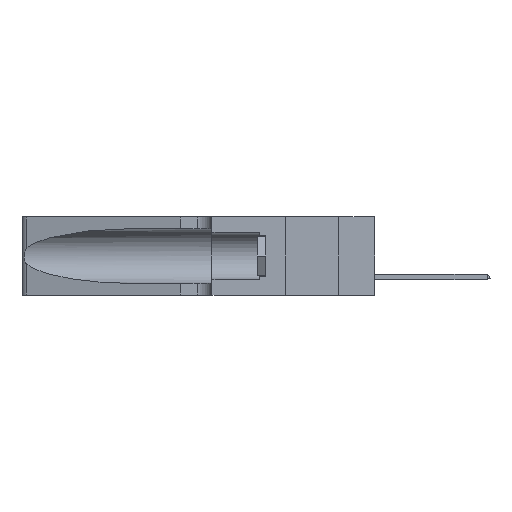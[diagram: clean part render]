
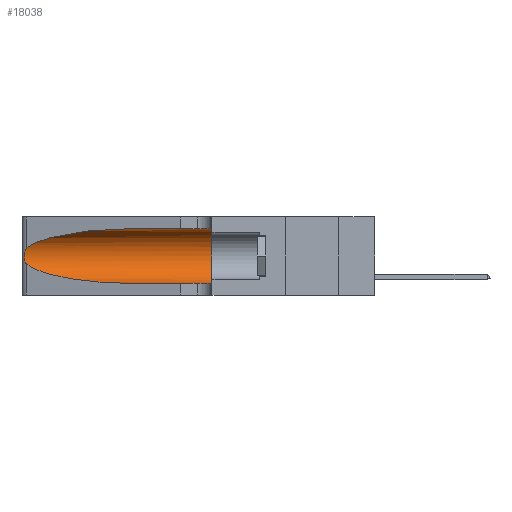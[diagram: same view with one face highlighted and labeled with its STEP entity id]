
A CAD part, left-side view. The second image highlights one B-rep face of the part: STEP entity #18038.
In plain terms, the highlighted cylindrical face has radius 3.308 mm (diameter 6.617 mm), a partial arc.
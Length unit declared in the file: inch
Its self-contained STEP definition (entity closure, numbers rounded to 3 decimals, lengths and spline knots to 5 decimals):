
#144 = CARTESIAN_POINT ( 'NONE',  ( 0.18966, 0.96281, 0.05475 ) ) ;
#435 = ORIENTED_EDGE ( 'NONE', *, *, #25085, .T. ) ;
#989 = CARTESIAN_POINT ( 'NONE',  ( 0.25787, 1.23484, 0.2124 ) ) ;
#1085 = CARTESIAN_POINT ( 'NONE',  ( 0.25487, 1.22718, 0.22369 ) ) ;
#1579 = DIRECTION ( 'NONE',  ( 0., -1., 0. ) ) ;
#2005 = ORIENTED_EDGE ( 'NONE', *, *, #19564, .T. ) ;
#2217 = CARTESIAN_POINT ( 'NONE',  ( 0.25487, 1.22718, 0.22369 ) ) ;
#2556 =( BOUNDED_CURVE ( )  B_SPLINE_CURVE ( 3, ( #8768, #8676, #17354, #2217 ),
 .UNSPECIFIED., .F., .F. ) 
 B_SPLINE_CURVE_WITH_KNOTS ( ( 4, 4 ),
 ( 1.5708, 2.84003 ),
 .UNSPECIFIED. ) 
 CURVE ( )  GEOMETRIC_REPRESENTATION_ITEM ( )  RATIONAL_B_SPLINE_CURVE ( ( 1., 0.87, 0.87, 1. ) ) 
 REPRESENTATION_ITEM ( '' )  );
#2606 = CARTESIAN_POINT ( 'NONE',  ( 0.1305, 0.35, 0.31525 ) ) ;
#3124 = CARTESIAN_POINT ( 'NONE',  ( 0.25487, 1.22718, 0.14631 ) ) ;
#3735 = CIRCLE ( 'NONE', #20630, 0.13025 ) ;
#3801 = CARTESIAN_POINT ( 'NONE',  ( 0.1305, 0.35, 0.05475 ) ) ;
#4142 = CARTESIAN_POINT ( 'NONE',  ( 0.1305, 1.61858, 0.05475 ) ) ;
#5543 = CARTESIAN_POINT ( 'NONE',  ( 0.26075, 1.23896, 0.19203 ) ) ;
#6054 = VECTOR ( 'NONE', #19007, 39.37008 ) ;
#6077 = EDGE_CURVE ( 'NONE', #18598, #22260, #2556, .T. ) ;
#6341 = CARTESIAN_POINT ( 'NONE',  ( 0.1305, 0.72297, 0.05475 ) ) ;
#6590 = CARTESIAN_POINT ( 'NONE',  ( 0.1305, 0.72297, 0.05475 ) ) ;
#6756 = CYLINDRICAL_SURFACE ( 'NONE', #26014, 0.13025 ) ;
#6841 = B_SPLINE_CURVE_WITH_KNOTS ( 'NONE', 3,
 ( #1085, #26986, #11624, #989, #11719, #15912, #5543, #13962, #26617, #7710, #26910, #9582, #18256, #3124 ),
 .UNSPECIFIED., .F., .F.,
 ( 4, 2, 2, 2, 2, 2, 4 ),
 ( 0., 0.00027, 0.00053, 0.00107, 0.0016, 0.00187, 0.00214 ),
 .UNSPECIFIED. ) ;
#7710 = CARTESIAN_POINT ( 'NONE',  ( 0.25856, 1.23593, 0.16098 ) ) ;
#7820 = CARTESIAN_POINT ( 'NONE',  ( 0.1305, 0.35, 0.185 ) ) ;
#8245 = EDGE_LOOP ( 'NONE', ( #21621, #435, #2005, #24810, #24538, #18217 ) ) ;
#8676 = CARTESIAN_POINT ( 'NONE',  ( 0.18966, 0.96281, 0.31525 ) ) ;
#8768 = CARTESIAN_POINT ( 'NONE',  ( 0.1305, 0.72297, 0.31525 ) ) ;
#9091 = LINE ( 'NONE', #4142, #6054 ) ;
#9095 = FACE_OUTER_BOUND ( 'NONE', #8245, .T. ) ;
#9199 = CARTESIAN_POINT ( 'NONE',  ( 0.25487, 1.22718, 0.14631 ) ) ;
#9582 = CARTESIAN_POINT ( 'NONE',  ( 0.25639, 1.23186, 0.15144 ) ) ;
#11074 = CARTESIAN_POINT ( 'NONE',  ( 0.2373, 1.15595, 0.08982 ) ) ;
#11624 = CARTESIAN_POINT ( 'NONE',  ( 0.25639, 1.23184, 0.21858 ) ) ;
#11719 = CARTESIAN_POINT ( 'NONE',  ( 0.25854, 1.2359, 0.20912 ) ) ;
#12083 = VERTEX_POINT ( 'NONE', #3801 ) ;
#12231 = VECTOR ( 'NONE', #19910, 39.37008 ) ;
#12979 = CARTESIAN_POINT ( 'NONE',  ( 0.25487, 1.22718, 0.22369 ) ) ;
#13149 = CARTESIAN_POINT ( 'NONE',  ( 0.25487, 1.22718, 0.14631 ) ) ;
#13962 = CARTESIAN_POINT ( 'NONE',  ( 0.26075, 1.23896, 0.178 ) ) ;
#14243 = LINE ( 'NONE', #15498, #12231 ) ;
#14373 = CARTESIAN_POINT ( 'NONE',  ( 0.1305, 1.61858, 0.185 ) ) ;
#15498 = CARTESIAN_POINT ( 'NONE',  ( 0.1305, 1.61858, 0.31525 ) ) ;
#15912 = CARTESIAN_POINT ( 'NONE',  ( 0.26018, 1.23835, 0.19895 ) ) ;
#16143 = EDGE_CURVE ( 'NONE', #18598, #23969, #14243, .T. ) ;
#17354 = CARTESIAN_POINT ( 'NONE',  ( 0.2373, 1.15595, 0.28018 ) ) ;
#18038 = ADVANCED_FACE ( 'NONE', ( #9095 ), #6756, .F. ) ;
#18217 = ORIENTED_EDGE ( 'NONE', *, *, #16143, .F. ) ;
#18256 = CARTESIAN_POINT ( 'NONE',  ( 0.25555, 1.22993, 0.14849 ) ) ;
#18598 = VERTEX_POINT ( 'NONE', #20969 ) ;
#18741 = DIRECTION ( 'NONE',  ( 0., 0., 1. ) ) ;
#19007 = DIRECTION ( 'NONE',  ( 0., -1., 0. ) ) ;
#19152 = EDGE_CURVE ( 'NONE', #23969, #12083, #3735, .T. ) ;
#19564 = EDGE_CURVE ( 'NONE', #26844, #26127, #24699, .T. ) ;
#19910 = DIRECTION ( 'NONE',  ( 0., -1., 0. ) ) ;
#20630 = AXIS2_PLACEMENT_3D ( 'NONE', #7820, #20818, #18741 ) ;
#20818 = DIRECTION ( 'NONE',  ( 0., 1., 0. ) ) ;
#20969 = CARTESIAN_POINT ( 'NONE',  ( 0.1305, 0.72297, 0.31525 ) ) ;
#21621 = ORIENTED_EDGE ( 'NONE', *, *, #6077, .T. ) ;
#22260 = VERTEX_POINT ( 'NONE', #12979 ) ;
#22933 = DIRECTION ( 'NONE',  ( 0., 0., -1. ) ) ;
#23969 = VERTEX_POINT ( 'NONE', #2606 ) ;
#24538 = ORIENTED_EDGE ( 'NONE', *, *, #19152, .F. ) ;
#24699 =( BOUNDED_CURVE ( )  B_SPLINE_CURVE ( 3, ( #13149, #11074, #144, #6590 ),
 .UNSPECIFIED., .F., .T. ) 
 B_SPLINE_CURVE_WITH_KNOTS ( ( 4, 4 ),
 ( 3.44316, 4.71239 ),
 .UNSPECIFIED. ) 
 CURVE ( )  GEOMETRIC_REPRESENTATION_ITEM ( )  RATIONAL_B_SPLINE_CURVE ( ( 1., 0.87, 0.87, 1. ) ) 
 REPRESENTATION_ITEM ( '' )  );
#24810 = ORIENTED_EDGE ( 'NONE', *, *, #27166, .T. ) ;
#25085 = EDGE_CURVE ( 'NONE', #22260, #26844, #6841, .T. ) ;
#26014 = AXIS2_PLACEMENT_3D ( 'NONE', #14373, #1579, #22933 ) ;
#26127 = VERTEX_POINT ( 'NONE', #6341 ) ;
#26617 = CARTESIAN_POINT ( 'NONE',  ( 0.26017, 1.23833, 0.17102 ) ) ;
#26844 = VERTEX_POINT ( 'NONE', #9199 ) ;
#26910 = CARTESIAN_POINT ( 'NONE',  ( 0.25789, 1.23486, 0.15765 ) ) ;
#26986 = CARTESIAN_POINT ( 'NONE',  ( 0.25555, 1.22994, 0.2215 ) ) ;
#27166 = EDGE_CURVE ( 'NONE', #26127, #12083, #9091, .T. ) ;
